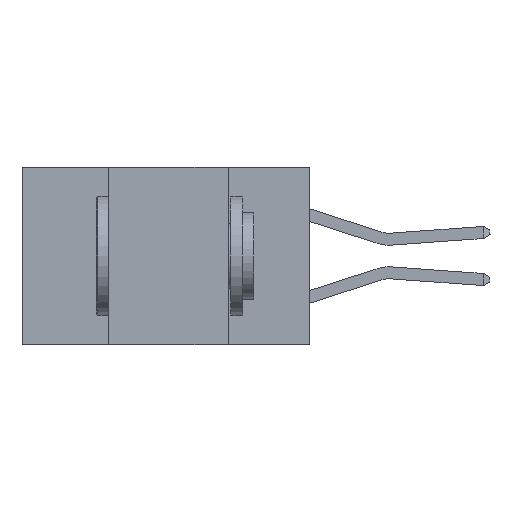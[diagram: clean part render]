
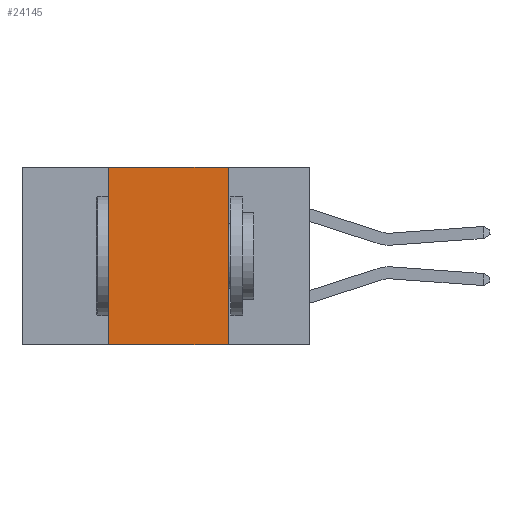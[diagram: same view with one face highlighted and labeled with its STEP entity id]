
A CAD part, left-side view. The second image highlights one B-rep face of the part: STEP entity #24145.
In plain terms, the highlighted planar face has unit normal (-1, 0, 0).
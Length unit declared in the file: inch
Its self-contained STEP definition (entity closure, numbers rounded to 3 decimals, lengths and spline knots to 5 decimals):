
#642 = DIRECTION ( 'NONE',  ( 0., 0., -1. ) ) ;
#965 = CARTESIAN_POINT ( 'NONE',  ( 0., 0.42, -0.37 ) ) ;
#1841 = VERTEX_POINT ( 'NONE', #9655 ) ;
#2144 = CARTESIAN_POINT ( 'NONE',  ( 0., 0.17, -0.37 ) ) ;
#3442 = VECTOR ( 'NONE', #24217, 39.37008 ) ;
#3538 = LINE ( 'NONE', #22919, #19133 ) ;
#4678 = LINE ( 'NONE', #23636, #20276 ) ;
#5718 = DIRECTION ( 'NONE',  ( 0., -1., 0. ) ) ;
#5839 = EDGE_CURVE ( 'NONE', #14535, #12419, #4678, .T. ) ;
#6508 = EDGE_CURVE ( 'NONE', #14535, #1841, #13585, .T. ) ;
#7744 = ORIENTED_EDGE ( 'NONE', *, *, #13793, .F. ) ;
#8120 = VECTOR ( 'NONE', #5718, 39.37008 ) ;
#8184 = FACE_OUTER_BOUND ( 'NONE', #18799, .T. ) ;
#8389 = VERTEX_POINT ( 'NONE', #8611 ) ;
#8611 = CARTESIAN_POINT ( 'NONE',  ( 0., 0.17, 0. ) ) ;
#9655 = CARTESIAN_POINT ( 'NONE',  ( 0., 0.42, 0. ) ) ;
#11491 = DIRECTION ( 'NONE',  ( 1., 0., 0. ) ) ;
#12419 = VERTEX_POINT ( 'NONE', #2144 ) ;
#13495 = LINE ( 'NONE', #25745, #8120 ) ;
#13585 = LINE ( 'NONE', #14086, #3442 ) ;
#13793 = EDGE_CURVE ( 'NONE', #8389, #12419, #3538, .T. ) ;
#14086 = CARTESIAN_POINT ( 'NONE',  ( 0., 0.42, -0.37 ) ) ;
#14535 = VERTEX_POINT ( 'NONE', #965 ) ;
#16321 = ORIENTED_EDGE ( 'NONE', *, *, #5839, .T. ) ;
#17554 = CARTESIAN_POINT ( 'NONE',  ( 0., 0.6, 0. ) ) ;
#18193 = EDGE_CURVE ( 'NONE', #1841, #8389, #13495, .T. ) ;
#18558 = ORIENTED_EDGE ( 'NONE', *, *, #18193, .F. ) ;
#18799 = EDGE_LOOP ( 'NONE', ( #7744, #18558, #25056, #16321 ) ) ;
#19133 = VECTOR ( 'NONE', #642, 39.37008 ) ;
#20276 = VECTOR ( 'NONE', #23727, 39.37008 ) ;
#22321 = AXIS2_PLACEMENT_3D ( 'NONE', #17554, #11491, #25519 ) ;
#22919 = CARTESIAN_POINT ( 'NONE',  ( 0., 0.17, -0.37 ) ) ;
#23571 = PLANE ( 'NONE',  #22321 ) ;
#23636 = CARTESIAN_POINT ( 'NONE',  ( 0., 0.6, -0.37 ) ) ;
#23727 = DIRECTION ( 'NONE',  ( 0., -1., 0. ) ) ;
#24145 = ADVANCED_FACE ( 'NONE', ( #8184 ), #23571, .F. ) ;
#24217 = DIRECTION ( 'NONE',  ( 0., 0., 1. ) ) ;
#25056 = ORIENTED_EDGE ( 'NONE', *, *, #6508, .F. ) ;
#25519 = DIRECTION ( 'NONE',  ( 0., 0., -1. ) ) ;
#25745 = CARTESIAN_POINT ( 'NONE',  ( 0., 0.6, 0. ) ) ;
